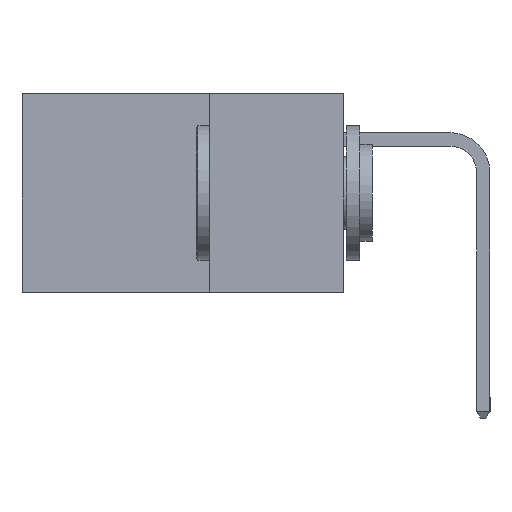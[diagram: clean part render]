
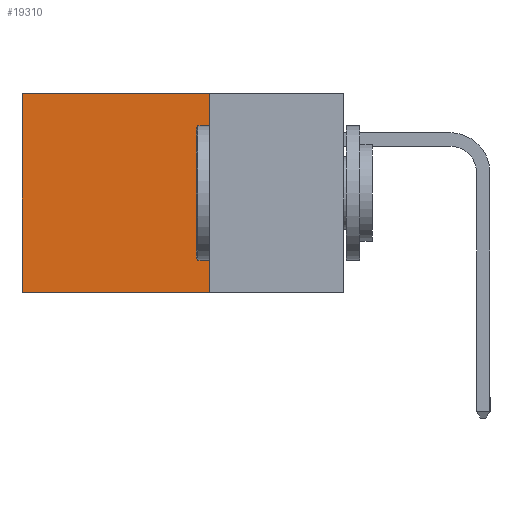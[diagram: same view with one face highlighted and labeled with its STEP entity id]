
A CAD part, left-side view. The second image highlights one B-rep face of the part: STEP entity #19310.
In plain terms, the highlighted planar face has unit normal (-1, 0, 0).
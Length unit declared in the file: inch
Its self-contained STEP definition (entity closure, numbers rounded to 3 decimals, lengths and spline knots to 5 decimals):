
#52 = ORIENTED_EDGE ( 'NONE', *, *, #16472, .F. ) ;
#239 = VECTOR ( 'NONE', #10425, 39.37008 ) ;
#559 = VERTEX_POINT ( 'NONE', #10712 ) ;
#751 = VERTEX_POINT ( 'NONE', #19597 ) ;
#1567 = LINE ( 'NONE', #18600, #9987 ) ;
#2593 = EDGE_LOOP ( 'NONE', ( #17821, #52, #9239, #21018 ) ) ;
#2926 = CARTESIAN_POINT ( 'NONE',  ( 0.2615, 0.6, -0.37 ) ) ;
#3087 = DIRECTION ( 'NONE',  ( 0., 0., -1. ) ) ;
#3294 = EDGE_CURVE ( 'NONE', #559, #4490, #14421, .T. ) ;
#4490 = VERTEX_POINT ( 'NONE', #9011 ) ;
#5970 = EDGE_CURVE ( 'NONE', #4490, #14055, #1567, .T. ) ;
#6005 = EDGE_CURVE ( 'NONE', #559, #751, #18039, .T. ) ;
#7151 = CARTESIAN_POINT ( 'NONE',  ( 0.2615, 0.25, 0. ) ) ;
#8890 = VECTOR ( 'NONE', #11513, 39.37008 ) ;
#9011 = CARTESIAN_POINT ( 'NONE',  ( 0.2615, 0.6, 0. ) ) ;
#9153 = CARTESIAN_POINT ( 'NONE',  ( 0.2615, 0.25, -0.37 ) ) ;
#9239 = ORIENTED_EDGE ( 'NONE', *, *, #6005, .F. ) ;
#9987 = VECTOR ( 'NONE', #17002, 39.37008 ) ;
#10425 = DIRECTION ( 'NONE',  ( 0., 1., 0. ) ) ;
#10712 = CARTESIAN_POINT ( 'NONE',  ( 0.2615, 0.25, 0. ) ) ;
#10913 = DIRECTION ( 'NONE',  ( 0., 1., 0. ) ) ;
#11513 = DIRECTION ( 'NONE',  ( 0., 0., -1. ) ) ;
#11928 = PLANE ( 'NONE',  #12765 ) ;
#12765 = AXIS2_PLACEMENT_3D ( 'NONE', #22050, #13662, #3087 ) ;
#12872 = CARTESIAN_POINT ( 'NONE',  ( 0.2615, 0.25, -0.37 ) ) ;
#13662 = DIRECTION ( 'NONE',  ( 1., 0., 0. ) ) ;
#14055 = VERTEX_POINT ( 'NONE', #2926 ) ;
#14421 = LINE ( 'NONE', #7151, #239 ) ;
#15474 = LINE ( 'NONE', #9153, #20498 ) ;
#16472 = EDGE_CURVE ( 'NONE', #751, #14055, #15474, .T. ) ;
#17002 = DIRECTION ( 'NONE',  ( 0., 0., -1. ) ) ;
#17040 = FACE_OUTER_BOUND ( 'NONE', #2593, .T. ) ;
#17821 = ORIENTED_EDGE ( 'NONE', *, *, #5970, .T. ) ;
#18039 = LINE ( 'NONE', #12872, #8890 ) ;
#18600 = CARTESIAN_POINT ( 'NONE',  ( 0.2615, 0.6, -0.37 ) ) ;
#19310 = ADVANCED_FACE ( 'NONE', ( #17040 ), #11928, .F. ) ;
#19597 = CARTESIAN_POINT ( 'NONE',  ( 0.2615, 0.25, -0.37 ) ) ;
#20498 = VECTOR ( 'NONE', #10913, 39.37008 ) ;
#21018 = ORIENTED_EDGE ( 'NONE', *, *, #3294, .T. ) ;
#22050 = CARTESIAN_POINT ( 'NONE',  ( 0.2615, 0.25, -0.37 ) ) ;
